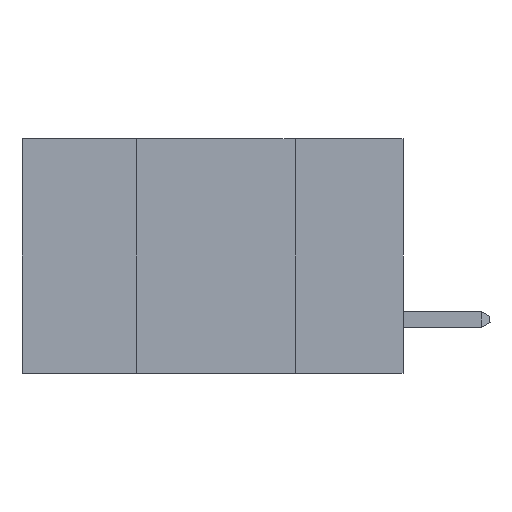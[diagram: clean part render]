
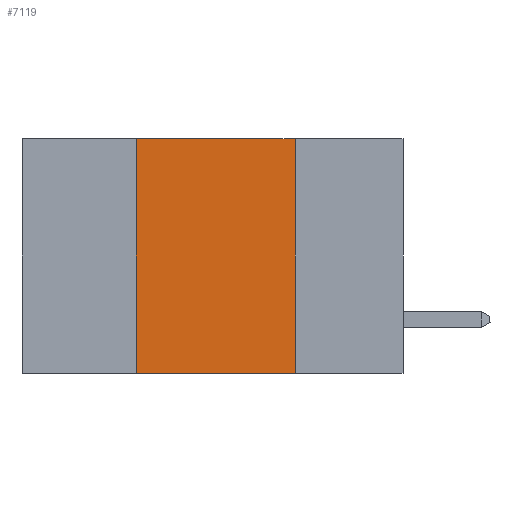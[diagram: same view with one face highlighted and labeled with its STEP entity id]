
A CAD part, left-side view. The second image highlights one B-rep face of the part: STEP entity #7119.
In plain terms, the highlighted planar face has unit normal (-1, 0, 0).
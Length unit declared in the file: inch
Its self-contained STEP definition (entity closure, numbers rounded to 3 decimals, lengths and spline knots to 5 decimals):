
#305 = VECTOR ( 'NONE', #26755, 39.37008 ) ;
#1021 = CARTESIAN_POINT ( 'NONE',  ( 0., 0.42, 0. ) ) ;
#1664 = LINE ( 'NONE', #24361, #2016 ) ;
#2016 = VECTOR ( 'NONE', #23276, 39.37008 ) ;
#3587 = ORIENTED_EDGE ( 'NONE', *, *, #10223, .F. ) ;
#3933 = CARTESIAN_POINT ( 'NONE',  ( 0., 0.6, 0. ) ) ;
#4967 = VERTEX_POINT ( 'NONE', #1021 ) ;
#5789 = LINE ( 'NONE', #3933, #305 ) ;
#5990 = FACE_OUTER_BOUND ( 'NONE', #25368, .T. ) ;
#6503 = LINE ( 'NONE', #22275, #6837 ) ;
#6837 = VECTOR ( 'NONE', #22717, 39.37008 ) ;
#7089 = DIRECTION ( 'NONE',  ( 1., 0., 0. ) ) ;
#7119 = ADVANCED_FACE ( 'NONE', ( #5990 ), #9086, .F. ) ;
#9086 = PLANE ( 'NONE',  #13186 ) ;
#9391 = ORIENTED_EDGE ( 'NONE', *, *, #25956, .F. ) ;
#10161 = EDGE_CURVE ( 'NONE', #14439, #20994, #20424, .T. ) ;
#10223 = EDGE_CURVE ( 'NONE', #4967, #24255, #5789, .T. ) ;
#12142 = CARTESIAN_POINT ( 'NONE',  ( 0., 0.42, -0.37 ) ) ;
#13186 = AXIS2_PLACEMENT_3D ( 'NONE', #13244, #7089, #16166 ) ;
#13244 = CARTESIAN_POINT ( 'NONE',  ( 0., 0.6, 0. ) ) ;
#14439 = VERTEX_POINT ( 'NONE', #12142 ) ;
#15497 = DIRECTION ( 'NONE',  ( 0., -1., 0. ) ) ;
#16166 = DIRECTION ( 'NONE',  ( 0., 0., -1. ) ) ;
#16586 = ORIENTED_EDGE ( 'NONE', *, *, #10161, .T. ) ;
#16686 = CARTESIAN_POINT ( 'NONE',  ( 0., 0.17, -0.37 ) ) ;
#17801 = VECTOR ( 'NONE', #15497, 39.37008 ) ;
#20424 = LINE ( 'NONE', #25634, #17801 ) ;
#20994 = VERTEX_POINT ( 'NONE', #16686 ) ;
#22275 = CARTESIAN_POINT ( 'NONE',  ( 0., 0.17, 0. ) ) ;
#22717 = DIRECTION ( 'NONE',  ( 0., 0., -1. ) ) ;
#22729 = EDGE_CURVE ( 'NONE', #14439, #4967, #1664, .T. ) ;
#22810 = ORIENTED_EDGE ( 'NONE', *, *, #22729, .F. ) ;
#23276 = DIRECTION ( 'NONE',  ( 0., 0., 1. ) ) ;
#24013 = CARTESIAN_POINT ( 'NONE',  ( 0., 0.17, 0. ) ) ;
#24255 = VERTEX_POINT ( 'NONE', #24013 ) ;
#24361 = CARTESIAN_POINT ( 'NONE',  ( 0., 0.42, 0. ) ) ;
#25368 = EDGE_LOOP ( 'NONE', ( #9391, #3587, #22810, #16586 ) ) ;
#25634 = CARTESIAN_POINT ( 'NONE',  ( 0., 0.6, -0.37 ) ) ;
#25956 = EDGE_CURVE ( 'NONE', #24255, #20994, #6503, .T. ) ;
#26755 = DIRECTION ( 'NONE',  ( 0., -1., 0. ) ) ;
